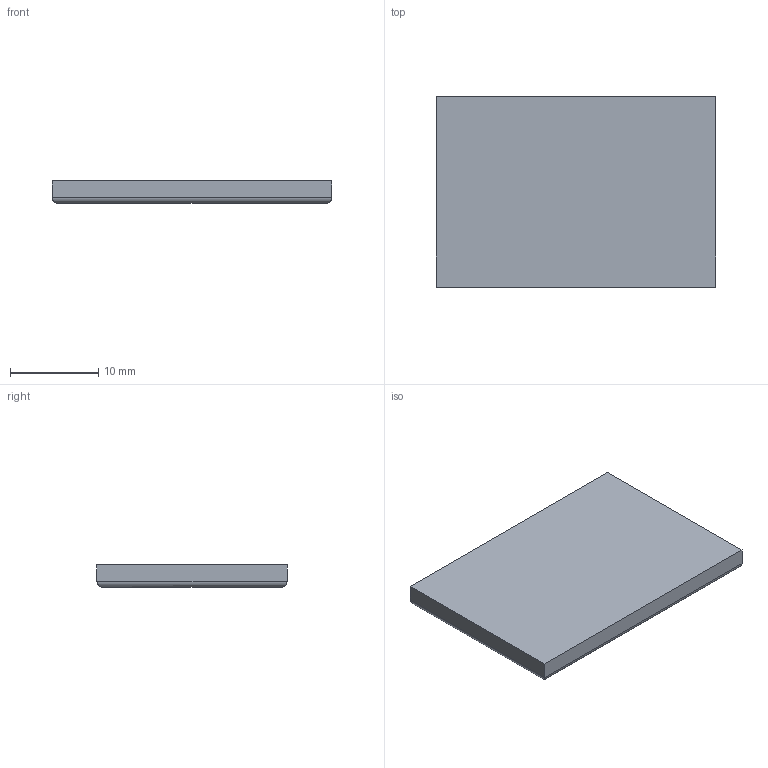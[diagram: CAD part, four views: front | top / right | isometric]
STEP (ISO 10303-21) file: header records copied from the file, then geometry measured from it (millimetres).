
FILE_DESCRIPTION (( 'STEP AP203' ), '1' );
FILE_NAME ('AF-WF-DP-PRT-001-SLDWRKS.STEP', '2020-07-21T18:37:00', ( '' ), ( '' ), 'SwSTEP 2.0', 'SolidWorks 2018', '' );
FILE_SCHEMA (( 'CONFIG_CONTROL_DESIGN' ));
Length unit declared in the file: inch
Products named in the file (1): AF-WF-DP-PRT-001-SLDWRKS
Bounding box: 31.75 x 21.59 x 2.54 mm (x, y, z)
Volume: 1732 mm3; surface area: 1612.6 mm2
Topology: 1 solids, 1 shells, 10 faces, 20 edges, 12 vertices
Faces by surface type: plane 6, cylinder 4
Entity records: 331 total; most frequent: CARTESIAN_POINT 55, ORIENTED_EDGE 40, DIRECTION 38, EDGE_CURVE 20, LINE 16, VECTOR 16, VERTEX_POINT 12, AXIS2_PLACEMENT_3D 11
